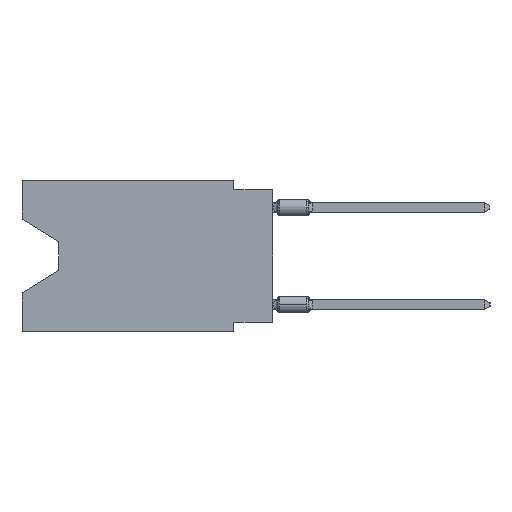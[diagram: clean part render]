
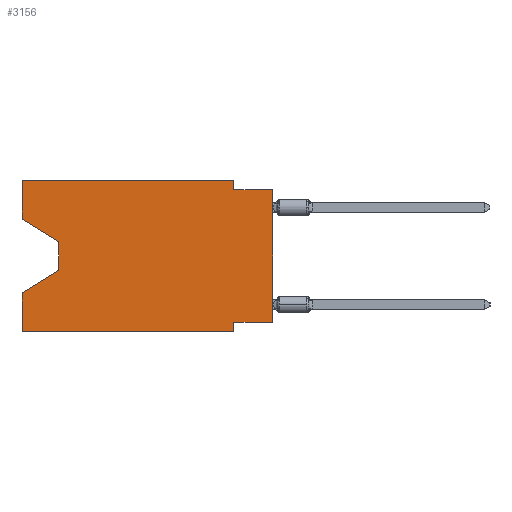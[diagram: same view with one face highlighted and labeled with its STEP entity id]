
A CAD part, left-side view. The second image highlights one B-rep face of the part: STEP entity #3156.
In plain terms, the highlighted planar face has unit normal (-1, 0, 0).
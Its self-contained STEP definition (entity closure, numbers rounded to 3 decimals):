
#125 = CARTESIAN_POINT ( 'NONE',  ( 0., 13.97, -4.013 ) ) ;
#303 = FACE_OUTER_BOUND ( 'NONE', #25404, .T. ) ;
#669 = VERTEX_POINT ( 'NONE', #695 ) ;
#695 = CARTESIAN_POINT ( 'NONE',  ( 0., 2.54, -0.635 ) ) ;
#767 = ORIENTED_EDGE ( 'NONE', *, *, #10522, .T. ) ;
#1650 = CARTESIAN_POINT ( 'NONE',  ( 0., 13.97, -4.013 ) ) ;
#1936 = DIRECTION ( 'NONE',  ( 0., 0., -1. ) ) ;
#2245 = LINE ( 'NONE', #30088, #10963 ) ;
#3156 = ADVANCED_FACE ( 'NONE', ( #303 ), #42235, .F. ) ;
#3860 = CARTESIAN_POINT ( 'NONE',  ( 0., 13.97, -5.893 ) ) ;
#4599 = CARTESIAN_POINT ( 'NONE',  ( 0., 16.383, 0. ) ) ;
#4775 = DIRECTION ( 'NONE',  ( 0., -1., 0. ) ) ;
#5272 = LINE ( 'NONE', #1650, #17777 ) ;
#5389 = EDGE_CURVE ( 'NONE', #28712, #41362, #48289, .T. ) ;
#5432 = CARTESIAN_POINT ( 'NONE',  ( 0., 2.54, 0. ) ) ;
#5632 = EDGE_CURVE ( 'NONE', #34761, #669, #46757, .T. ) ;
#5803 = VERTEX_POINT ( 'NONE', #3860 ) ;
#6001 = DIRECTION ( 'NONE',  ( 1., 0., 0. ) ) ;
#6342 = LINE ( 'NONE', #24305, #6790 ) ;
#6609 = DIRECTION ( 'NONE',  ( 0., 0., -1. ) ) ;
#6782 = EDGE_CURVE ( 'NONE', #28712, #29668, #16906, .T. ) ;
#6790 = VECTOR ( 'NONE', #51286, 1000. ) ;
#7244 = CARTESIAN_POINT ( 'NONE',  ( 0., 0., 0. ) ) ;
#7371 = EDGE_CURVE ( 'NONE', #669, #41362, #18553, .T. ) ;
#7803 = DIRECTION ( 'NONE',  ( 0., 0.855, -0.519 ) ) ;
#8130 = VERTEX_POINT ( 'NONE', #125 ) ;
#9667 = LINE ( 'NONE', #37521, #56638 ) ;
#9722 = CARTESIAN_POINT ( 'NONE',  ( 0., 16.383, 0. ) ) ;
#10187 = ORIENTED_EDGE ( 'NONE', *, *, #6782, .F. ) ;
#10522 = EDGE_CURVE ( 'NONE', #18152, #26992, #58651, .T. ) ;
#10963 = VECTOR ( 'NONE', #16041, 1000. ) ;
#11319 = EDGE_CURVE ( 'NONE', #29668, #26992, #2245, .T. ) ;
#13002 = CARTESIAN_POINT ( 'NONE',  ( 0., 0., -9.271 ) ) ;
#13082 = ORIENTED_EDGE ( 'NONE', *, *, #5389, .T. ) ;
#13125 = DIRECTION ( 'NONE',  ( 0., -1., 0. ) ) ;
#14375 = DIRECTION ( 'NONE',  ( 0., 0., -1. ) ) ;
#14437 = CARTESIAN_POINT ( 'NONE',  ( 0., 2.54, -9.906 ) ) ;
#14507 = ORIENTED_EDGE ( 'NONE', *, *, #21053, .F. ) ;
#14650 = CARTESIAN_POINT ( 'NONE',  ( 0., 16.383, -9.906 ) ) ;
#16041 = DIRECTION ( 'NONE',  ( 0., 0., -1. ) ) ;
#16597 = VECTOR ( 'NONE', #17922, 1000. ) ;
#16906 = LINE ( 'NONE', #13002, #54738 ) ;
#17665 = EDGE_CURVE ( 'NONE', #39421, #8130, #6342, .T. ) ;
#17777 = VECTOR ( 'NONE', #1936, 1000. ) ;
#17922 = DIRECTION ( 'NONE',  ( 0., 0., 1. ) ) ;
#17949 = VECTOR ( 'NONE', #23755, 1000. ) ;
#18152 = VERTEX_POINT ( 'NONE', #14650 ) ;
#18197 = ORIENTED_EDGE ( 'NONE', *, *, #7371, .F. ) ;
#18553 = LINE ( 'NONE', #27528, #51919 ) ;
#19039 = CARTESIAN_POINT ( 'NONE',  ( 0., 2.54, -9.271 ) ) ;
#19249 = VECTOR ( 'NONE', #43782, 1000. ) ;
#19555 = DIRECTION ( 'NONE',  ( 0., 0., 1. ) ) ;
#21053 = EDGE_CURVE ( 'NONE', #18152, #49306, #54159, .T. ) ;
#23076 = CARTESIAN_POINT ( 'NONE',  ( 0., 16.383, 0. ) ) ;
#23161 = ORIENTED_EDGE ( 'NONE', *, *, #42357, .T. ) ;
#23755 = DIRECTION ( 'NONE',  ( 0., -1., 0. ) ) ;
#24268 = CARTESIAN_POINT ( 'NONE',  ( 0., 0., -9.271 ) ) ;
#24305 = CARTESIAN_POINT ( 'NONE',  ( 0., 16.383, -2.546 ) ) ;
#25404 = EDGE_LOOP ( 'NONE', ( #53811, #30174, #23161, #14507, #767, #40460, #10187, #13082, #18197, #28911, #48942, #44579 ) ) ;
#26377 = CARTESIAN_POINT ( 'NONE',  ( 0., 13.97, -5.893 ) ) ;
#26992 = VERTEX_POINT ( 'NONE', #14437 ) ;
#27528 = CARTESIAN_POINT ( 'NONE',  ( 0., 0., -0.635 ) ) ;
#27658 = AXIS2_PLACEMENT_3D ( 'NONE', #23076, #6001, #14375 ) ;
#27875 = VECTOR ( 'NONE', #6609, 1000. ) ;
#28154 = VERTEX_POINT ( 'NONE', #31017 ) ;
#28712 = VERTEX_POINT ( 'NONE', #24268 ) ;
#28911 = ORIENTED_EDGE ( 'NONE', *, *, #5632, .F. ) ;
#29668 = VERTEX_POINT ( 'NONE', #19039 ) ;
#30088 = CARTESIAN_POINT ( 'NONE',  ( 0., 2.54, -9.906 ) ) ;
#30174 = ORIENTED_EDGE ( 'NONE', *, *, #37878, .T. ) ;
#30976 = VECTOR ( 'NONE', #7803, 1000. ) ;
#31017 = CARTESIAN_POINT ( 'NONE',  ( 0., 16.383, 0. ) ) ;
#34761 = VERTEX_POINT ( 'NONE', #35282 ) ;
#35282 = CARTESIAN_POINT ( 'NONE',  ( 0., 2.54, 0. ) ) ;
#36181 = CARTESIAN_POINT ( 'NONE',  ( 0., 16.383, -9.906 ) ) ;
#37521 = CARTESIAN_POINT ( 'NONE',  ( 0., 16.383, 0. ) ) ;
#37878 = EDGE_CURVE ( 'NONE', #8130, #5803, #5272, .T. ) ;
#38599 = CARTESIAN_POINT ( 'NONE',  ( 0., 0., -0.635 ) ) ;
#39421 = VERTEX_POINT ( 'NONE', #53982 ) ;
#40460 = ORIENTED_EDGE ( 'NONE', *, *, #11319, .F. ) ;
#41362 = VERTEX_POINT ( 'NONE', #38599 ) ;
#42235 = PLANE ( 'NONE',  #27658 ) ;
#42357 = EDGE_CURVE ( 'NONE', #5803, #49306, #44051, .T. ) ;
#43782 = DIRECTION ( 'NONE',  ( 0., 0., 1. ) ) ;
#44051 = LINE ( 'NONE', #26377, #30976 ) ;
#44579 = ORIENTED_EDGE ( 'NONE', *, *, #55272, .F. ) ;
#46519 = LINE ( 'NONE', #4599, #17949 ) ;
#46592 = CARTESIAN_POINT ( 'NONE',  ( 0., 16.383, -7.36 ) ) ;
#46757 = LINE ( 'NONE', #5432, #27875 ) ;
#48289 = LINE ( 'NONE', #7244, #19249 ) ;
#48942 = ORIENTED_EDGE ( 'NONE', *, *, #49691, .F. ) ;
#49306 = VERTEX_POINT ( 'NONE', #46592 ) ;
#49691 = EDGE_CURVE ( 'NONE', #28154, #34761, #46519, .T. ) ;
#51286 = DIRECTION ( 'NONE',  ( 0., -0.855, -0.519 ) ) ;
#51919 = VECTOR ( 'NONE', #4775, 1000. ) ;
#53448 = DIRECTION ( 'NONE',  ( 0., 1., 0. ) ) ;
#53811 = ORIENTED_EDGE ( 'NONE', *, *, #17665, .T. ) ;
#53982 = CARTESIAN_POINT ( 'NONE',  ( 0., 16.383, -2.546 ) ) ;
#54159 = LINE ( 'NONE', #9722, #16597 ) ;
#54738 = VECTOR ( 'NONE', #53448, 1000. ) ;
#55272 = EDGE_CURVE ( 'NONE', #39421, #28154, #9667, .T. ) ;
#56638 = VECTOR ( 'NONE', #19555, 1000. ) ;
#56811 = VECTOR ( 'NONE', #13125, 1000. ) ;
#58651 = LINE ( 'NONE', #36181, #56811 ) ;
